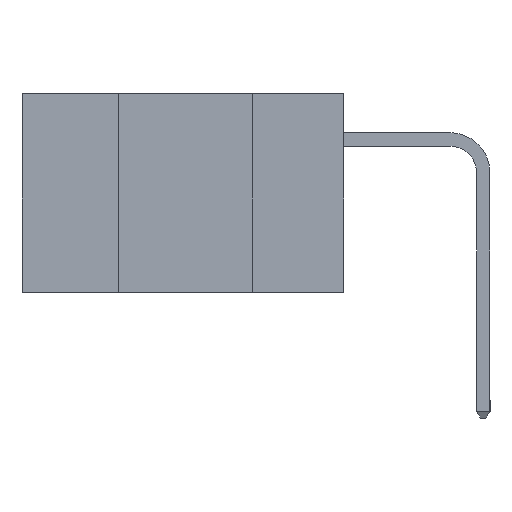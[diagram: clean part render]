
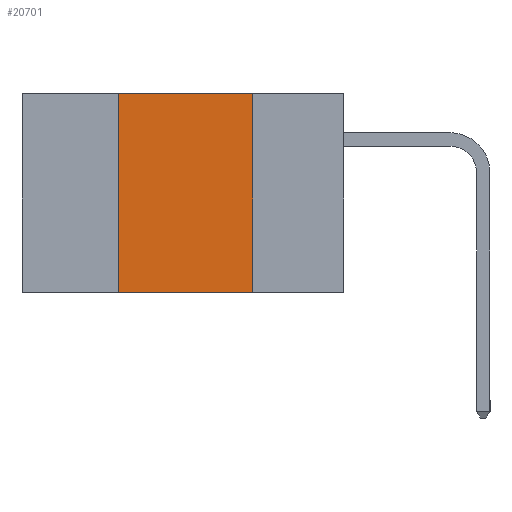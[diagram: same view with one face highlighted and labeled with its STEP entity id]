
A CAD part, left-side view. The second image highlights one B-rep face of the part: STEP entity #20701.
In plain terms, the highlighted planar face has unit normal (-1, 0, 0).
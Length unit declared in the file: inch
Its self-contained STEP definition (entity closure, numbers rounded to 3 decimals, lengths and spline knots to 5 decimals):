
#370 = ORIENTED_EDGE ( 'NONE', *, *, #25277, .F. ) ;
#868 = ORIENTED_EDGE ( 'NONE', *, *, #17894, .F. ) ;
#1088 = VERTEX_POINT ( 'NONE', #23290 ) ;
#1110 = ORIENTED_EDGE ( 'NONE', *, *, #17403, .F. ) ;
#1193 = ORIENTED_EDGE ( 'NONE', *, *, #23529, .T. ) ;
#3683 = PLANE ( 'NONE',  #7982 ) ;
#5076 = LINE ( 'NONE', #12763, #25128 ) ;
#5718 = DIRECTION ( 'NONE',  ( 0., 0., -1. ) ) ;
#6985 = VECTOR ( 'NONE', #9107, 39.37008 ) ;
#7132 = CARTESIAN_POINT ( 'NONE',  ( 0., 0.42, -0.37 ) ) ;
#7656 = VECTOR ( 'NONE', #13172, 39.37008 ) ;
#7982 = AXIS2_PLACEMENT_3D ( 'NONE', #15492, #17406, #5718 ) ;
#9107 = DIRECTION ( 'NONE',  ( 0., 0., 1. ) ) ;
#11072 = CARTESIAN_POINT ( 'NONE',  ( 0., 0.42, 0. ) ) ;
#11237 = CARTESIAN_POINT ( 'NONE',  ( 0., 0.42, -0.37 ) ) ;
#12190 = LINE ( 'NONE', #7132, #6985 ) ;
#12763 = CARTESIAN_POINT ( 'NONE',  ( 0., 0.6, 0. ) ) ;
#13094 = FACE_OUTER_BOUND ( 'NONE', #19657, .T. ) ;
#13172 = DIRECTION ( 'NONE',  ( 0., 0., -1. ) ) ;
#15465 = DIRECTION ( 'NONE',  ( 0., -1., 0. ) ) ;
#15492 = CARTESIAN_POINT ( 'NONE',  ( 0., 0.6, 0. ) ) ;
#15591 = VERTEX_POINT ( 'NONE', #24851 ) ;
#15714 = LINE ( 'NONE', #23123, #20204 ) ;
#16176 = VERTEX_POINT ( 'NONE', #11072 ) ;
#17403 = EDGE_CURVE ( 'NONE', #22499, #16176, #12190, .T. ) ;
#17406 = DIRECTION ( 'NONE',  ( 1., 0., 0. ) ) ;
#17894 = EDGE_CURVE ( 'NONE', #16176, #1088, #5076, .T. ) ;
#18999 = CARTESIAN_POINT ( 'NONE',  ( 0., 0.17, -0.37 ) ) ;
#19657 = EDGE_LOOP ( 'NONE', ( #370, #868, #1110, #1193 ) ) ;
#20204 = VECTOR ( 'NONE', #15465, 39.37008 ) ;
#20701 = ADVANCED_FACE ( 'NONE', ( #13094 ), #3683, .F. ) ;
#22489 = DIRECTION ( 'NONE',  ( 0., -1., 0. ) ) ;
#22499 = VERTEX_POINT ( 'NONE', #11237 ) ;
#23123 = CARTESIAN_POINT ( 'NONE',  ( 0., 0.6, -0.37 ) ) ;
#23290 = CARTESIAN_POINT ( 'NONE',  ( 0., 0.17, 0. ) ) ;
#23529 = EDGE_CURVE ( 'NONE', #22499, #15591, #15714, .T. ) ;
#23715 = LINE ( 'NONE', #18999, #7656 ) ;
#24851 = CARTESIAN_POINT ( 'NONE',  ( 0., 0.17, -0.37 ) ) ;
#25128 = VECTOR ( 'NONE', #22489, 39.37008 ) ;
#25277 = EDGE_CURVE ( 'NONE', #1088, #15591, #23715, .T. ) ;
